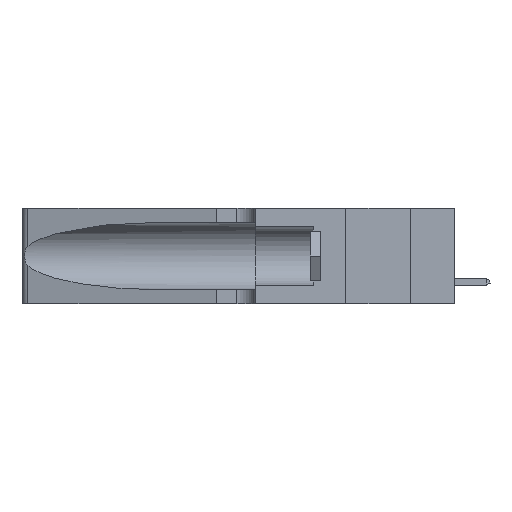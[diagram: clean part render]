
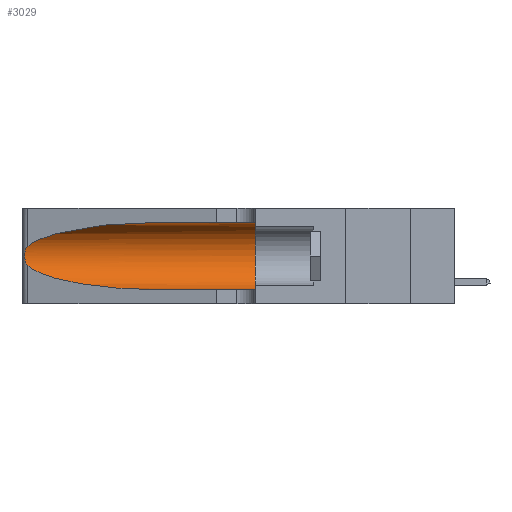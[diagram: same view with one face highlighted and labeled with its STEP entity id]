
A CAD part, left-side view. The second image highlights one B-rep face of the part: STEP entity #3029.
In plain terms, the highlighted cylindrical face has radius 3.308 mm (diameter 6.617 mm), a partial arc.
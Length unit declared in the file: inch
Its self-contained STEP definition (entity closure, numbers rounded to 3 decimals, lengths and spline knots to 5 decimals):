
#832 = CARTESIAN_POINT ( 'NONE',  ( 0.25639, 1.23186, 0.15144 ) ) ;
#910 = CARTESIAN_POINT ( 'NONE',  ( 0.25555, 1.22993, 0.14849 ) ) ;
#1041 = CARTESIAN_POINT ( 'NONE',  ( 0.25487, 1.22718, 0.22369 ) ) ;
#1313 = LINE ( 'NONE', #6524, #20445 ) ;
#1667 = DIRECTION ( 'NONE',  ( 0., 0., 1. ) ) ;
#2049 = CYLINDRICAL_SURFACE ( 'NONE', #14222, 0.13025 ) ;
#2210 = EDGE_CURVE ( 'NONE', #7140, #21106, #3266, .T. ) ;
#2251 = AXIS2_PLACEMENT_3D ( 'NONE', #12807, #13031, #1667 ) ;
#2647 = ORIENTED_EDGE ( 'NONE', *, *, #10406, .T. ) ;
#2666 = FACE_OUTER_BOUND ( 'NONE', #7880, .T. ) ;
#3029 = ADVANCED_FACE ( 'NONE', ( #2666 ), #2049, .F. ) ;
#3266 = CIRCLE ( 'NONE', #2251, 0.13025 ) ;
#3335 = ORIENTED_EDGE ( 'NONE', *, *, #9060, .T. ) ;
#3567 =( BOUNDED_CURVE ( )  B_SPLINE_CURVE ( 3, ( #5936, #14226, #17787, #23138 ),
 .UNSPECIFIED., .F., .F. ) 
 B_SPLINE_CURVE_WITH_KNOTS ( ( 4, 4 ),
 ( 3.44316, 4.71239 ),
 .UNSPECIFIED. ) 
 CURVE ( )  GEOMETRIC_REPRESENTATION_ITEM ( )  RATIONAL_B_SPLINE_CURVE ( ( 1., 0.87, 0.87, 1. ) ) 
 REPRESENTATION_ITEM ( '' )  );
#4123 = ORIENTED_EDGE ( 'NONE', *, *, #19944, .T. ) ;
#4247 = CARTESIAN_POINT ( 'NONE',  ( 0.1305, 0.35, 0.31525 ) ) ;
#4481 = CARTESIAN_POINT ( 'NONE',  ( 0.26018, 1.23835, 0.19895 ) ) ;
#5193 = VERTEX_POINT ( 'NONE', #9606 ) ;
#5936 = CARTESIAN_POINT ( 'NONE',  ( 0.25487, 1.22718, 0.14631 ) ) ;
#6336 = CARTESIAN_POINT ( 'NONE',  ( 0.26075, 1.23896, 0.178 ) ) ;
#6343 = CARTESIAN_POINT ( 'NONE',  ( 0.1305, 1.61858, 0.185 ) ) ;
#6424 = DIRECTION ( 'NONE',  ( 0., -1., 0. ) ) ;
#6518 = B_SPLINE_CURVE_WITH_KNOTS ( 'NONE', 3,
 ( #21013, #11875, #19226, #22960, #15617, #4481, #17464, #6336, #12028, #10115, #23048, #832, #910, #13907 ),
 .UNSPECIFIED., .F., .F.,
 ( 4, 2, 2, 2, 2, 2, 4 ),
 ( 0., 0.00027, 0.00053, 0.00107, 0.0016, 0.00187, 0.00214 ),
 .UNSPECIFIED. ) ;
#6524 = CARTESIAN_POINT ( 'NONE',  ( 0.1305, 1.61858, 0.31525 ) ) ;
#6864 = LINE ( 'NONE', #21987, #12973 ) ;
#6938 = CARTESIAN_POINT ( 'NONE',  ( 0.1305, 0.72297, 0.31525 ) ) ;
#7087 = ORIENTED_EDGE ( 'NONE', *, *, #2210, .F. ) ;
#7140 = VERTEX_POINT ( 'NONE', #4247 ) ;
#7880 = EDGE_LOOP ( 'NONE', ( #3335, #4123, #2647, #12253, #7087, #10944 ) ) ;
#8716 = DIRECTION ( 'NONE',  ( 0., 0., -1. ) ) ;
#9060 = EDGE_CURVE ( 'NONE', #14075, #5193, #17831, .T. ) ;
#9606 = CARTESIAN_POINT ( 'NONE',  ( 0.25487, 1.22718, 0.22369 ) ) ;
#10115 = CARTESIAN_POINT ( 'NONE',  ( 0.25856, 1.23593, 0.16098 ) ) ;
#10406 = EDGE_CURVE ( 'NONE', #16097, #11638, #3567, .T. ) ;
#10944 = ORIENTED_EDGE ( 'NONE', *, *, #21711, .F. ) ;
#11638 = VERTEX_POINT ( 'NONE', #15909 ) ;
#11875 = CARTESIAN_POINT ( 'NONE',  ( 0.25555, 1.22994, 0.2215 ) ) ;
#12028 = CARTESIAN_POINT ( 'NONE',  ( 0.26017, 1.23833, 0.17102 ) ) ;
#12253 = ORIENTED_EDGE ( 'NONE', *, *, #18666, .T. ) ;
#12807 = CARTESIAN_POINT ( 'NONE',  ( 0.1305, 0.35, 0.185 ) ) ;
#12973 = VECTOR ( 'NONE', #22309, 39.37008 ) ;
#13031 = DIRECTION ( 'NONE',  ( 0., 1., 0. ) ) ;
#13285 = CARTESIAN_POINT ( 'NONE',  ( 0.1305, 0.72297, 0.31525 ) ) ;
#13782 = DIRECTION ( 'NONE',  ( 0., -1., 0. ) ) ;
#13907 = CARTESIAN_POINT ( 'NONE',  ( 0.25487, 1.22718, 0.14631 ) ) ;
#14075 = VERTEX_POINT ( 'NONE', #13285 ) ;
#14178 = CARTESIAN_POINT ( 'NONE',  ( 0.2373, 1.15595, 0.28018 ) ) ;
#14222 = AXIS2_PLACEMENT_3D ( 'NONE', #6343, #6424, #8716 ) ;
#14226 = CARTESIAN_POINT ( 'NONE',  ( 0.2373, 1.15595, 0.08982 ) ) ;
#15617 = CARTESIAN_POINT ( 'NONE',  ( 0.25854, 1.2359, 0.20912 ) ) ;
#15745 = CARTESIAN_POINT ( 'NONE',  ( 0.25487, 1.22718, 0.14631 ) ) ;
#15909 = CARTESIAN_POINT ( 'NONE',  ( 0.1305, 0.72297, 0.05475 ) ) ;
#16097 = VERTEX_POINT ( 'NONE', #15745 ) ;
#17464 = CARTESIAN_POINT ( 'NONE',  ( 0.26075, 1.23896, 0.19203 ) ) ;
#17787 = CARTESIAN_POINT ( 'NONE',  ( 0.18966, 0.96281, 0.05475 ) ) ;
#17831 =( BOUNDED_CURVE ( )  B_SPLINE_CURVE ( 3, ( #6938, #19841, #14178, #1041 ),
 .UNSPECIFIED., .F., .T. ) 
 B_SPLINE_CURVE_WITH_KNOTS ( ( 4, 4 ),
 ( 1.5708, 2.84003 ),
 .UNSPECIFIED. ) 
 CURVE ( )  GEOMETRIC_REPRESENTATION_ITEM ( )  RATIONAL_B_SPLINE_CURVE ( ( 1., 0.87, 0.87, 1. ) ) 
 REPRESENTATION_ITEM ( '' )  );
#18666 = EDGE_CURVE ( 'NONE', #11638, #21106, #6864, .T. ) ;
#19226 = CARTESIAN_POINT ( 'NONE',  ( 0.25639, 1.23184, 0.21858 ) ) ;
#19841 = CARTESIAN_POINT ( 'NONE',  ( 0.18966, 0.96281, 0.31525 ) ) ;
#19944 = EDGE_CURVE ( 'NONE', #5193, #16097, #6518, .T. ) ;
#20445 = VECTOR ( 'NONE', #13782, 39.37008 ) ;
#21013 = CARTESIAN_POINT ( 'NONE',  ( 0.25487, 1.22718, 0.22369 ) ) ;
#21106 = VERTEX_POINT ( 'NONE', #22379 ) ;
#21711 = EDGE_CURVE ( 'NONE', #14075, #7140, #1313, .T. ) ;
#21987 = CARTESIAN_POINT ( 'NONE',  ( 0.1305, 1.61858, 0.05475 ) ) ;
#22309 = DIRECTION ( 'NONE',  ( 0., -1., 0. ) ) ;
#22379 = CARTESIAN_POINT ( 'NONE',  ( 0.1305, 0.35, 0.05475 ) ) ;
#22960 = CARTESIAN_POINT ( 'NONE',  ( 0.25787, 1.23484, 0.2124 ) ) ;
#23048 = CARTESIAN_POINT ( 'NONE',  ( 0.25789, 1.23486, 0.15765 ) ) ;
#23138 = CARTESIAN_POINT ( 'NONE',  ( 0.1305, 0.72297, 0.05475 ) ) ;
